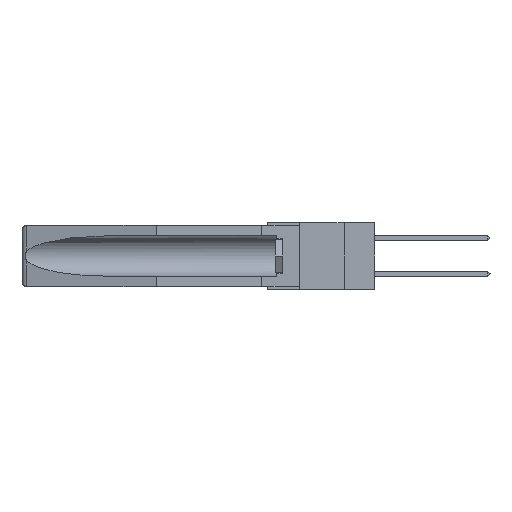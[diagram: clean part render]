
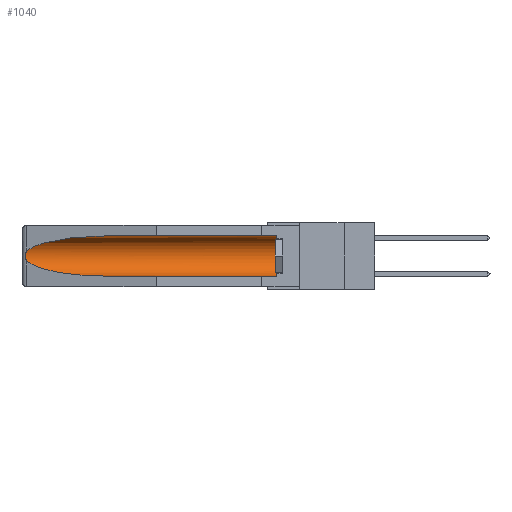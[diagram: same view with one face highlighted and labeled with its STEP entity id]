
A CAD part, left-side view. The second image highlights one B-rep face of the part: STEP entity #1040.
In plain terms, the highlighted cylindrical face has radius 2.857 mm (diameter 5.715 mm), a partial arc.
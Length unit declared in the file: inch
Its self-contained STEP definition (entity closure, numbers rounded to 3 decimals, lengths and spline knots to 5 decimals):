
#1040 = ADVANCED_FACE ( 'NONE', ( #15051 ), #13600, .F. ) ;
#1080 = CARTESIAN_POINT ( 'NONE',  ( 0.155, 1.07973, -0.059 ) ) ;
#1117 = CARTESIAN_POINT ( 'NONE',  ( 0.26537, 1.52718, -0.19328 ) ) ;
#1132 = CARTESIAN_POINT ( 'NONE',  ( 0.2675, 1.53308, -0.17534 ) ) ;
#1571 = CARTESIAN_POINT ( 'NONE',  ( 0.155, -0.30754, -0.059 ) ) ;
#1781 = EDGE_CURVE ( 'NONE', #10046, #20403, #13589, .T. ) ;
#1812 = ORIENTED_EDGE ( 'NONE', *, *, #18526, .T. ) ;
#1860 = CARTESIAN_POINT ( 'NONE',  ( 0.25451, 1.48313, -0.24835 ) ) ;
#3394 = ORIENTED_EDGE ( 'NONE', *, *, #18115, .T. ) ;
#3461 = DIRECTION ( 'NONE',  ( 0., 1., 0. ) ) ;
#4019 = CARTESIAN_POINT ( 'NONE',  ( 0.26537, 1.52718, -0.14972 ) ) ;
#4257 = CARTESIAN_POINT ( 'NONE',  ( 0.21114, 1.30732, -0.059 ) ) ;
#4775 = CARTESIAN_POINT ( 'NONE',  ( 0.2673, 1.53269, -0.17917 ) ) ;
#4774 = DIRECTION ( 'NONE',  ( 0., 1., 0. ) ) ;
#5043 = CARTESIAN_POINT ( 'NONE',  ( 0.26537, 1.52718, -0.14972 ) ) ;
#5969 = AXIS2_PLACEMENT_3D ( 'NONE', #15616, #11704, #10014 ) ;
#6457 = CARTESIAN_POINT ( 'NONE',  ( 0.155, 0.126, -0.284 ) ) ;
#6601 = CARTESIAN_POINT ( 'NONE',  ( 0.2675, 1.53308, -0.16763 ) ) ;
#6821 = VECTOR ( 'NONE', #3461, 39.37008 ) ;
#7564 =( BOUNDED_CURVE ( )  B_SPLINE_CURVE ( 3, ( #22166, #4257, #13099, #4019 ),
 .UNSPECIFIED., .F., .T. ) 
 B_SPLINE_CURVE_WITH_KNOTS ( ( 4, 4 ),
 ( 4.71239, 6.08839 ),
 .UNSPECIFIED. ) 
 CURVE ( )  GEOMETRIC_REPRESENTATION_ITEM ( )  RATIONAL_B_SPLINE_CURVE ( ( 1., 0.848, 0.848, 1. ) ) 
 REPRESENTATION_ITEM ( '' )  );
#7905 = EDGE_CURVE ( 'NONE', #22266, #8582, #15939, .T. ) ;
#7969 = LINE ( 'NONE', #1571, #6821 ) ;
#7997 = CARTESIAN_POINT ( 'NONE',  ( 0.155, 0.126, -0.1715 ) ) ;
#8582 = VERTEX_POINT ( 'NONE', #21969 ) ;
#9057 = CARTESIAN_POINT ( 'NONE',  ( 0.26537, 1.52718, -0.19328 ) ) ;
#9537 = CARTESIAN_POINT ( 'NONE',  ( 0.155, 1.07973, -0.284 ) ) ;
#9758 =( BOUNDED_CURVE ( )  B_SPLINE_CURVE ( 3, ( #9057, #1860, #12984, #21718 ),
 .UNSPECIFIED., .F., .F. ) 
 B_SPLINE_CURVE_WITH_KNOTS ( ( 4, 4 ),
 ( 0.1948, 1.5708 ),
 .UNSPECIFIED. ) 
 CURVE ( )  GEOMETRIC_REPRESENTATION_ITEM ( )  RATIONAL_B_SPLINE_CURVE ( ( 1., 0.848, 0.848, 1. ) ) 
 REPRESENTATION_ITEM ( '' )  );
#10014 = DIRECTION ( 'NONE',  ( 0., 0., 1. ) ) ;
#10046 = VERTEX_POINT ( 'NONE', #5043 ) ;
#10589 = CARTESIAN_POINT ( 'NONE',  ( 0.26537, 1.52718, -0.19328 ) ) ;
#11051 = EDGE_CURVE ( 'NONE', #15942, #10046, #7564, .T. ) ;
#11442 = ORIENTED_EDGE ( 'NONE', *, *, #7905, .T. ) ;
#11660 = ORIENTED_EDGE ( 'NONE', *, *, #11051, .T. ) ;
#11704 = DIRECTION ( 'NONE',  ( 0., 1., 0. ) ) ;
#11866 = AXIS2_PLACEMENT_3D ( 'NONE', #7997, #22428, #18631 ) ;
#12984 = CARTESIAN_POINT ( 'NONE',  ( 0.21114, 1.30732, -0.284 ) ) ;
#13099 = CARTESIAN_POINT ( 'NONE',  ( 0.25451, 1.48313, -0.09465 ) ) ;
#13589 = B_SPLINE_CURVE_WITH_KNOTS ( 'NONE', 3,
 ( #14110, #21099, #15934, #21405, #6601, #1132, #4775, #19375, #17838, #10589 ),
 .UNSPECIFIED., .F., .F.,
 ( 4, 2, 2, 2, 4 ),
 ( 0., 0.00029, 0.00058, 0.00087, 0.00117 ),
 .UNSPECIFIED. ) ;
#13600 = CYLINDRICAL_SURFACE ( 'NONE', #5969, 0.1125 ) ;
#14068 = VECTOR ( 'NONE', #4774, 39.37008 ) ;
#14110 = CARTESIAN_POINT ( 'NONE',  ( 0.26537, 1.52718, -0.14972 ) ) ;
#15051 = FACE_OUTER_BOUND ( 'NONE', #17889, .T. ) ;
#15616 = CARTESIAN_POINT ( 'NONE',  ( 0.155, -0.30754, -0.1715 ) ) ;
#15649 = EDGE_CURVE ( 'NONE', #22266, #18144, #22885, .T. ) ;
#15934 = CARTESIAN_POINT ( 'NONE',  ( 0.26654, 1.53092, -0.15636 ) ) ;
#15933 = CARTESIAN_POINT ( 'NONE',  ( 0.155, -0.30754, -0.284 ) ) ;
#15939 = CIRCLE ( 'NONE', #11866, 0.1125 ) ;
#15942 = VERTEX_POINT ( 'NONE', #1080 ) ;
#17838 = CARTESIAN_POINT ( 'NONE',  ( 0.26597, 1.5296, -0.19026 ) ) ;
#17889 = EDGE_LOOP ( 'NONE', ( #11660, #18530, #3394, #21928, #11442, #1812 ) ) ;
#18115 = EDGE_CURVE ( 'NONE', #20403, #18144, #9758, .T. ) ;
#18144 = VERTEX_POINT ( 'NONE', #9537 ) ;
#18526 = EDGE_CURVE ( 'NONE', #8582, #15942, #7969, .T. ) ;
#18530 = ORIENTED_EDGE ( 'NONE', *, *, #1781, .T. ) ;
#18631 = DIRECTION ( 'NONE',  ( 0., 0., 1. ) ) ;
#19375 = CARTESIAN_POINT ( 'NONE',  ( 0.26655, 1.53094, -0.18657 ) ) ;
#20403 = VERTEX_POINT ( 'NONE', #1117 ) ;
#21099 = CARTESIAN_POINT ( 'NONE',  ( 0.26597, 1.52961, -0.15275 ) ) ;
#21405 = CARTESIAN_POINT ( 'NONE',  ( 0.2673, 1.5327, -0.16383 ) ) ;
#21718 = CARTESIAN_POINT ( 'NONE',  ( 0.155, 1.07973, -0.284 ) ) ;
#21928 = ORIENTED_EDGE ( 'NONE', *, *, #15649, .F. ) ;
#21969 = CARTESIAN_POINT ( 'NONE',  ( 0.155, 0.126, -0.059 ) ) ;
#22166 = CARTESIAN_POINT ( 'NONE',  ( 0.155, 1.07973, -0.059 ) ) ;
#22266 = VERTEX_POINT ( 'NONE', #6457 ) ;
#22428 = DIRECTION ( 'NONE',  ( 0., -1., 0. ) ) ;
#22885 = LINE ( 'NONE', #15933, #14068 ) ;
